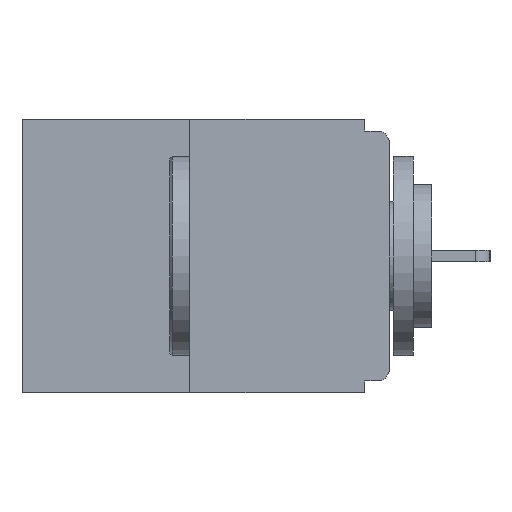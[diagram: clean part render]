
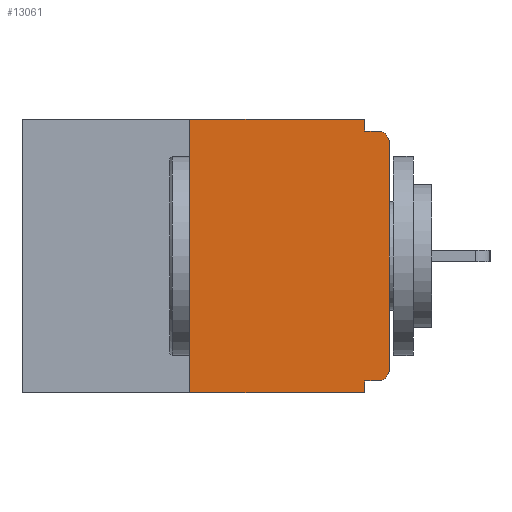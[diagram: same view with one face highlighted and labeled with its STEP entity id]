
A CAD part, left-side view. The second image highlights one B-rep face of the part: STEP entity #13061.
In plain terms, the highlighted planar face has unit normal (-1, 0, 0).
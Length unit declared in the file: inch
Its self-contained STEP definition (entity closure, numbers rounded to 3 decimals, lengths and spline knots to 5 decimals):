
#31 = LINE ( 'NONE', #13805, #7406 ) ;
#86 = CARTESIAN_POINT ( 'NONE',  ( 0., 0.015, -0.313 ) ) ;
#262 = VECTOR ( 'NONE', #13725, 39.37008 ) ;
#288 = ORIENTED_EDGE ( 'NONE', *, *, #10561, .F. ) ;
#551 = AXIS2_PLACEMENT_3D ( 'NONE', #3669, #10565, #7165 ) ;
#894 = CARTESIAN_POINT ( 'NONE',  ( 0., 0.25, 0. ) ) ;
#919 = VERTEX_POINT ( 'NONE', #9768 ) ;
#1093 = CARTESIAN_POINT ( 'NONE',  ( 0., 0.46, 0. ) ) ;
#1114 = DIRECTION ( 'NONE',  ( 0., 1., 0. ) ) ;
#1136 = CARTESIAN_POINT ( 'NONE',  ( 0., 0., -0.313 ) ) ;
#1318 = DIRECTION ( 'NONE',  ( 0., 0., -1. ) ) ;
#1510 = VECTOR ( 'NONE', #9493, 39.37008 ) ;
#1652 = VERTEX_POINT ( 'NONE', #7033 ) ;
#1900 = ORIENTED_EDGE ( 'NONE', *, *, #7561, .F. ) ;
#2199 = LINE ( 'NONE', #894, #9892 ) ;
#3003 = VERTEX_POINT ( 'NONE', #12404 ) ;
#3197 = LINE ( 'NONE', #6678, #10945 ) ;
#3398 = CARTESIAN_POINT ( 'NONE',  ( 0., 0.015, -0.015 ) ) ;
#3417 = DIRECTION ( 'NONE',  ( 0., 0., -1. ) ) ;
#3523 = PLANE ( 'NONE',  #12687 ) ;
#3669 = CARTESIAN_POINT ( 'NONE',  ( 0., 0.015, -0.03 ) ) ;
#3927 = EDGE_CURVE ( 'NONE', #5173, #13969, #3197, .T. ) ;
#3960 = CIRCLE ( 'NONE', #11891, 0.015 ) ;
#4342 = EDGE_CURVE ( 'NONE', #13582, #4421, #10136, .T. ) ;
#4421 = VERTEX_POINT ( 'NONE', #3398 ) ;
#4487 = EDGE_CURVE ( 'NONE', #14442, #1652, #14076, .T. ) ;
#4783 = DIRECTION ( 'NONE',  ( -1., 0., 0. ) ) ;
#4836 = EDGE_CURVE ( 'NONE', #919, #12931, #8340, .T. ) ;
#4991 = ORIENTED_EDGE ( 'NONE', *, *, #8264, .T. ) ;
#5173 = VERTEX_POINT ( 'NONE', #1136 ) ;
#5280 = ORIENTED_EDGE ( 'NONE', *, *, #10885, .F. ) ;
#5339 = DIRECTION ( 'NONE',  ( 0., 0., -1. ) ) ;
#5578 = EDGE_CURVE ( 'NONE', #6610, #3003, #15118, .T. ) ;
#6089 = CARTESIAN_POINT ( 'NONE',  ( 0., 0.25, -0.343 ) ) ;
#6610 = VERTEX_POINT ( 'NONE', #6089 ) ;
#6678 = CARTESIAN_POINT ( 'NONE',  ( 0., 0., 0. ) ) ;
#7033 = CARTESIAN_POINT ( 'NONE',  ( 0., 0.031, -0.328 ) ) ;
#7045 = CARTESIAN_POINT ( 'NONE',  ( 0., 0., -0.328 ) ) ;
#7157 = VECTOR ( 'NONE', #14802, 39.37008 ) ;
#7165 = DIRECTION ( 'NONE',  ( 0., 0., -1. ) ) ;
#7346 = ORIENTED_EDGE ( 'NONE', *, *, #7852, .T. ) ;
#7406 = VECTOR ( 'NONE', #3417, 39.37008 ) ;
#7471 = VECTOR ( 'NONE', #5339, 39.37008 ) ;
#7561 = EDGE_CURVE ( 'NONE', #12931, #13582, #7744, .T. ) ;
#7744 = LINE ( 'NONE', #14796, #7471 ) ;
#7852 = EDGE_CURVE ( 'NONE', #14442, #5173, #3960, .T. ) ;
#8063 = DIRECTION ( 'NONE',  ( 0., 0., 1. ) ) ;
#8264 = EDGE_CURVE ( 'NONE', #13969, #4421, #8683, .T. ) ;
#8340 = LINE ( 'NONE', #1093, #1510 ) ;
#8387 = VECTOR ( 'NONE', #1114, 39.37008 ) ;
#8683 = CIRCLE ( 'NONE', #551, 0.015 ) ;
#9399 = CARTESIAN_POINT ( 'NONE',  ( 0., 0.46, 0. ) ) ;
#9493 = DIRECTION ( 'NONE',  ( 0., -1., 0. ) ) ;
#9768 = CARTESIAN_POINT ( 'NONE',  ( 0., 0.25, 0. ) ) ;
#9892 = VECTOR ( 'NONE', #13788, 39.37008 ) ;
#10136 = LINE ( 'NONE', #12715, #7157 ) ;
#10515 = DIRECTION ( 'NONE',  ( 0., 0., -1. ) ) ;
#10556 = ORIENTED_EDGE ( 'NONE', *, *, #4836, .F. ) ;
#10561 = EDGE_CURVE ( 'NONE', #1652, #3003, #31, .T. ) ;
#10565 = DIRECTION ( 'NONE',  ( -1., 0., 0. ) ) ;
#10676 = ORIENTED_EDGE ( 'NONE', *, *, #4342, .F. ) ;
#10879 = DIRECTION ( 'NONE',  ( 1., 0., 0. ) ) ;
#10885 = EDGE_CURVE ( 'NONE', #6610, #919, #2199, .T. ) ;
#10945 = VECTOR ( 'NONE', #8063, 39.37008 ) ;
#11891 = AXIS2_PLACEMENT_3D ( 'NONE', #86, #4783, #10515 ) ;
#12404 = CARTESIAN_POINT ( 'NONE',  ( 0., 0.031, -0.343 ) ) ;
#12603 = EDGE_LOOP ( 'NONE', ( #10556, #5280, #14469, #288, #14279, #7346, #14399, #4991, #10676, #1900 ) ) ;
#12687 = AXIS2_PLACEMENT_3D ( 'NONE', #9399, #10879, #1318 ) ;
#12715 = CARTESIAN_POINT ( 'NONE',  ( 0., 0., -0.015 ) ) ;
#12931 = VERTEX_POINT ( 'NONE', #13828 ) ;
#13061 = ADVANCED_FACE ( 'NONE', ( #14127 ), #3523, .F. ) ;
#13181 = CARTESIAN_POINT ( 'NONE',  ( 0., 0.015, -0.328 ) ) ;
#13208 = CARTESIAN_POINT ( 'NONE',  ( 0., 0.031, -0.015 ) ) ;
#13582 = VERTEX_POINT ( 'NONE', #13208 ) ;
#13725 = DIRECTION ( 'NONE',  ( 0., -1., 0. ) ) ;
#13788 = DIRECTION ( 'NONE',  ( 0., 0., 1. ) ) ;
#13805 = CARTESIAN_POINT ( 'NONE',  ( 0., 0.031, -0.343 ) ) ;
#13828 = CARTESIAN_POINT ( 'NONE',  ( 0., 0.031, 0. ) ) ;
#13942 = CARTESIAN_POINT ( 'NONE',  ( 0., 0.46, -0.343 ) ) ;
#13969 = VERTEX_POINT ( 'NONE', #14329 ) ;
#14076 = LINE ( 'NONE', #7045, #8387 ) ;
#14127 = FACE_OUTER_BOUND ( 'NONE', #12603, .T. ) ;
#14279 = ORIENTED_EDGE ( 'NONE', *, *, #4487, .F. ) ;
#14329 = CARTESIAN_POINT ( 'NONE',  ( 0., 0., -0.03 ) ) ;
#14399 = ORIENTED_EDGE ( 'NONE', *, *, #3927, .T. ) ;
#14442 = VERTEX_POINT ( 'NONE', #13181 ) ;
#14469 = ORIENTED_EDGE ( 'NONE', *, *, #5578, .T. ) ;
#14796 = CARTESIAN_POINT ( 'NONE',  ( 0., 0.031, 0. ) ) ;
#14802 = DIRECTION ( 'NONE',  ( 0., -1., 0. ) ) ;
#15118 = LINE ( 'NONE', #13942, #262 ) ;
